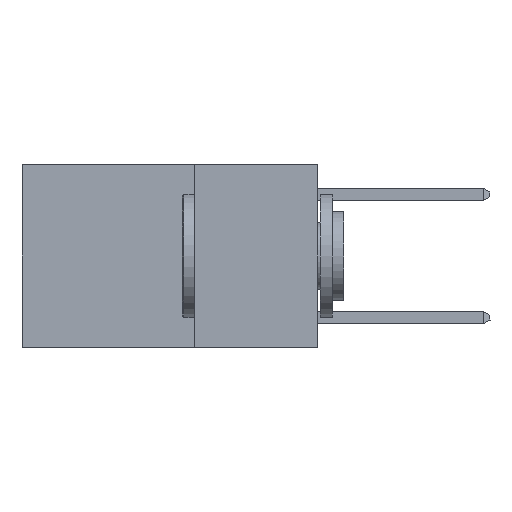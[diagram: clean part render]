
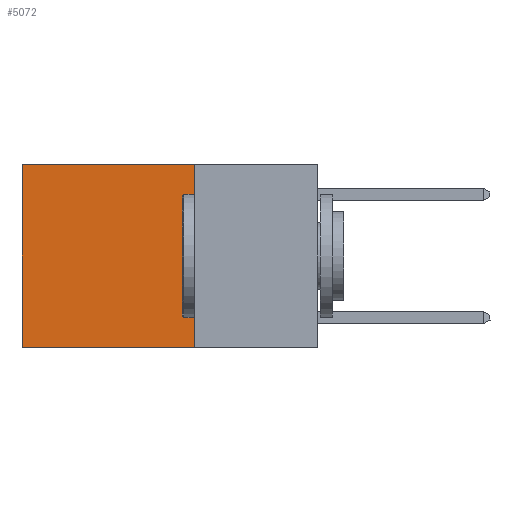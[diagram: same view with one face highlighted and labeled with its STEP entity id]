
A CAD part, left-side view. The second image highlights one B-rep face of the part: STEP entity #5072.
In plain terms, the highlighted planar face has unit normal (-1, 0, 0).
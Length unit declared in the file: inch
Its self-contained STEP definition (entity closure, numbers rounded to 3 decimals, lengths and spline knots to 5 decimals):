
#349 = ORIENTED_EDGE ( 'NONE', *, *, #1061, .F. ) ;
#506 = VERTEX_POINT ( 'NONE', #11657 ) ;
#851 = ORIENTED_EDGE ( 'NONE', *, *, #8206, .F. ) ;
#933 = CARTESIAN_POINT ( 'NONE',  ( 0.2625, 0.6, 0. ) ) ;
#1061 = EDGE_CURVE ( 'NONE', #506, #1230, #6034, .T. ) ;
#1134 = AXIS2_PLACEMENT_3D ( 'NONE', #4464, #5377, #11982 ) ;
#1230 = VERTEX_POINT ( 'NONE', #7828 ) ;
#2108 = ORIENTED_EDGE ( 'NONE', *, *, #5204, .T. ) ;
#3498 = LINE ( 'NONE', #6101, #5684 ) ;
#3783 = VECTOR ( 'NONE', #7470, 39.37008 ) ;
#4464 = CARTESIAN_POINT ( 'NONE',  ( 0.2625, 0.25, 0. ) ) ;
#4540 = VERTEX_POINT ( 'NONE', #11006 ) ;
#5072 = ADVANCED_FACE ( 'NONE', ( #5225 ), #9096, .F. ) ;
#5204 = EDGE_CURVE ( 'NONE', #4540, #1230, #8141, .T. ) ;
#5225 = FACE_OUTER_BOUND ( 'NONE', #8148, .T. ) ;
#5358 = ORIENTED_EDGE ( 'NONE', *, *, #6333, .T. ) ;
#5377 = DIRECTION ( 'NONE',  ( 1., 0., 0. ) ) ;
#5475 = VECTOR ( 'NONE', #9825, 39.37008 ) ;
#5684 = VECTOR ( 'NONE', #9836, 39.37008 ) ;
#6034 = LINE ( 'NONE', #9843, #5475 ) ;
#6101 = CARTESIAN_POINT ( 'NONE',  ( 0.2625, 0.25, 0. ) ) ;
#6333 = EDGE_CURVE ( 'NONE', #6335, #4540, #3498, .T. ) ;
#6335 = VERTEX_POINT ( 'NONE', #6971 ) ;
#6372 = DIRECTION ( 'NONE',  ( 0., 0., -1. ) ) ;
#6971 = CARTESIAN_POINT ( 'NONE',  ( 0.2625, 0.25, 0. ) ) ;
#7200 = VECTOR ( 'NONE', #6372, 39.37008 ) ;
#7470 = DIRECTION ( 'NONE',  ( 0., 0., -1. ) ) ;
#7828 = CARTESIAN_POINT ( 'NONE',  ( 0.2625, 0.6, -0.37 ) ) ;
#8141 = LINE ( 'NONE', #933, #3783 ) ;
#8148 = EDGE_LOOP ( 'NONE', ( #2108, #349, #851, #5358 ) ) ;
#8206 = EDGE_CURVE ( 'NONE', #6335, #506, #11997, .T. ) ;
#9096 = PLANE ( 'NONE',  #1134 ) ;
#9825 = DIRECTION ( 'NONE',  ( 0., 1., 0. ) ) ;
#9836 = DIRECTION ( 'NONE',  ( 0., 1., 0. ) ) ;
#9843 = CARTESIAN_POINT ( 'NONE',  ( 0.2625, 0.25, -0.37 ) ) ;
#11006 = CARTESIAN_POINT ( 'NONE',  ( 0.2625, 0.6, 0. ) ) ;
#11657 = CARTESIAN_POINT ( 'NONE',  ( 0.2625, 0.25, -0.37 ) ) ;
#11982 = DIRECTION ( 'NONE',  ( 0., 0., -1. ) ) ;
#11997 = LINE ( 'NONE', #12062, #7200 ) ;
#12062 = CARTESIAN_POINT ( 'NONE',  ( 0.2625, 0.25, 0. ) ) ;
